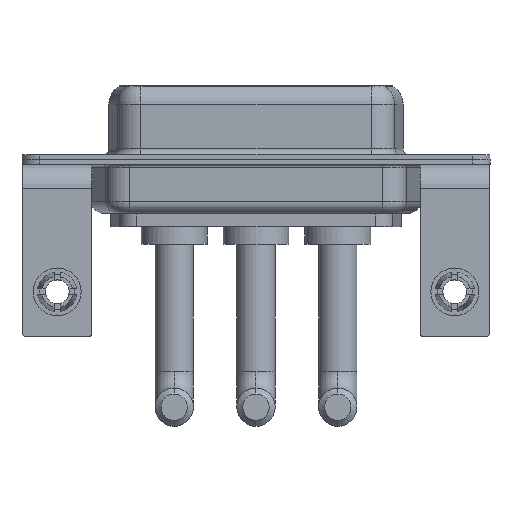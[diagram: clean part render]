
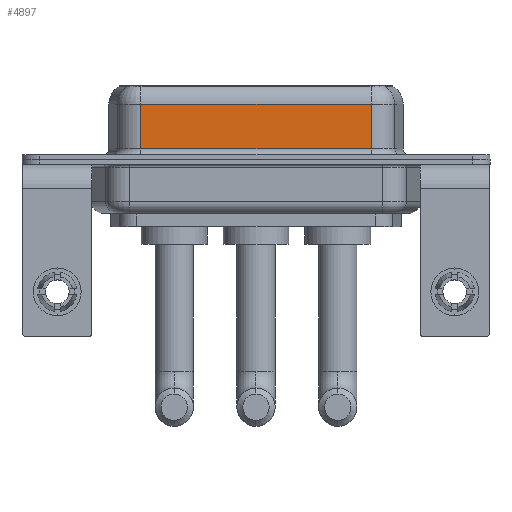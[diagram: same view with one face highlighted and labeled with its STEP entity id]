
A CAD part, front view. The second image highlights one B-rep face of the part: STEP entity #4897.
In plain terms, the highlighted planar face has unit normal (0, -1, 0).
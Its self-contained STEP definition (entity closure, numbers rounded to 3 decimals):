
#46 = VERTEX_POINT ( 'NONE', #12088 ) ;
#245 = EDGE_CURVE ( 'NONE', #4167, #46, #3890, .T. ) ;
#1520 = DIRECTION ( 'NONE',  ( 0., 0., -1. ) ) ;
#1841 = ORIENTED_EDGE ( 'NONE', *, *, #3617, .F. ) ;
#2296 = EDGE_CURVE ( 'NONE', #7626, #4167, #3695, .T. ) ;
#2505 = CARTESIAN_POINT ( 'NONE',  ( 7.013, -3.95, 0.9 ) ) ;
#2849 = CARTESIAN_POINT ( 'NONE',  ( 26.287, -3.95, 6.4 ) ) ;
#3617 = EDGE_CURVE ( 'NONE', #10045, #46, #13116, .T. ) ;
#3695 = LINE ( 'NONE', #11726, #10719 ) ;
#3890 = LINE ( 'NONE', #7307, #8958 ) ;
#4167 = VERTEX_POINT ( 'NONE', #2505 ) ;
#4897 = ADVANCED_FACE ( 'NONE', ( #10600 ), #5026, .F. ) ;
#5026 = PLANE ( 'NONE',  #9638 ) ;
#5307 = VECTOR ( 'NONE', #8790, 1000. ) ;
#5488 = ORIENTED_EDGE ( 'NONE', *, *, #2296, .T. ) ;
#6063 = VECTOR ( 'NONE', #9693, 1000. ) ;
#6210 = DIRECTION ( 'NONE',  ( 0., 1., 0. ) ) ;
#6641 = LINE ( 'NONE', #10947, #5307 ) ;
#7088 = ORIENTED_EDGE ( 'NONE', *, *, #14150, .T. ) ;
#7307 = CARTESIAN_POINT ( 'NONE',  ( 26.287, -3.95, 0.9 ) ) ;
#7626 = VERTEX_POINT ( 'NONE', #8158 ) ;
#8158 = CARTESIAN_POINT ( 'NONE',  ( 7.013, -3.95, 4.65 ) ) ;
#8303 = EDGE_LOOP ( 'NONE', ( #1841, #7088, #5488, #10877 ) ) ;
#8790 = DIRECTION ( 'NONE',  ( -1., 0., 0. ) ) ;
#8958 = VECTOR ( 'NONE', #11916, 1000. ) ;
#9536 = CARTESIAN_POINT ( 'NONE',  ( 26.287, -3.95, 4.65 ) ) ;
#9638 = AXIS2_PLACEMENT_3D ( 'NONE', #2849, #6210, #10742 ) ;
#9693 = DIRECTION ( 'NONE',  ( 0., 0., -1. ) ) ;
#10045 = VERTEX_POINT ( 'NONE', #9536 ) ;
#10600 = FACE_OUTER_BOUND ( 'NONE', #8303, .T. ) ;
#10719 = VECTOR ( 'NONE', #1520, 1000. ) ;
#10742 = DIRECTION ( 'NONE',  ( 0., 0., 1. ) ) ;
#10802 = CARTESIAN_POINT ( 'NONE',  ( 26.287, -3.95, 6.4 ) ) ;
#10877 = ORIENTED_EDGE ( 'NONE', *, *, #245, .T. ) ;
#10947 = CARTESIAN_POINT ( 'NONE',  ( 26.287, -3.95, 4.65 ) ) ;
#11726 = CARTESIAN_POINT ( 'NONE',  ( 7.013, -3.95, 6.4 ) ) ;
#11916 = DIRECTION ( 'NONE',  ( 1., 0., 0. ) ) ;
#12088 = CARTESIAN_POINT ( 'NONE',  ( 26.287, -3.95, 0.9 ) ) ;
#13116 = LINE ( 'NONE', #10802, #6063 ) ;
#14150 = EDGE_CURVE ( 'NONE', #10045, #7626, #6641, .T. ) ;
